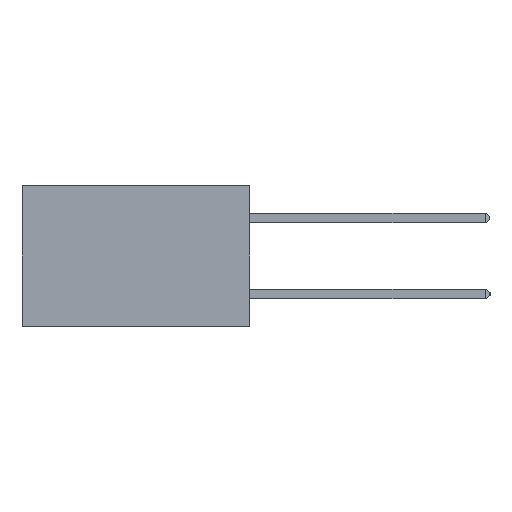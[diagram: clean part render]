
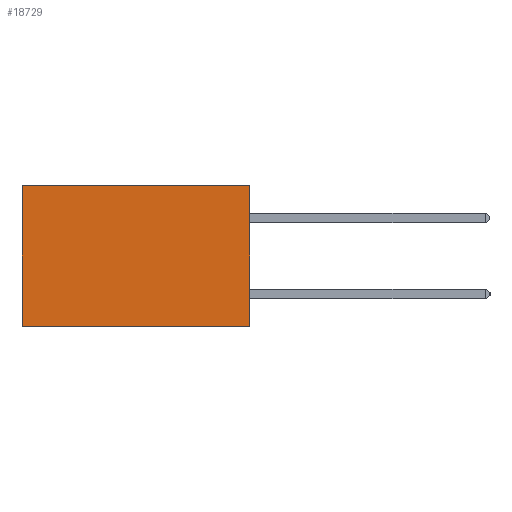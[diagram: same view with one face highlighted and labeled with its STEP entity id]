
A CAD part, left-side view. The second image highlights one B-rep face of the part: STEP entity #18729.
In plain terms, the highlighted planar face has unit normal (-1, 0, 0).
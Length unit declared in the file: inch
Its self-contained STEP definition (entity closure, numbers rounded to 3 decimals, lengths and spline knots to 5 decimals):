
#870 = DIRECTION ( 'NONE',  ( 0., 0., -1. ) ) ;
#1429 = VERTEX_POINT ( 'NONE', #18514 ) ;
#1780 = ORIENTED_EDGE ( 'NONE', *, *, #9348, .T. ) ;
#2032 = VECTOR ( 'NONE', #22287, 39.37008 ) ;
#2166 = VERTEX_POINT ( 'NONE', #12702 ) ;
#5112 = VECTOR ( 'NONE', #22371, 39.37008 ) ;
#5744 = LINE ( 'NONE', #7700, #2032 ) ;
#6310 = CARTESIAN_POINT ( 'NONE',  ( 0.2875, 0., 0. ) ) ;
#6389 = DIRECTION ( 'NONE',  ( 1., 0., 0. ) ) ;
#6594 = CARTESIAN_POINT ( 'NONE',  ( 0.2875, 0., -0.37 ) ) ;
#7700 = CARTESIAN_POINT ( 'NONE',  ( 0.2875, 0., 0. ) ) ;
#7823 = ORIENTED_EDGE ( 'NONE', *, *, #16398, .F. ) ;
#8543 = LINE ( 'NONE', #6594, #5112 ) ;
#9080 = VERTEX_POINT ( 'NONE', #19997 ) ;
#9171 = EDGE_CURVE ( 'NONE', #9080, #1429, #5744, .T. ) ;
#9348 = EDGE_CURVE ( 'NONE', #1429, #2166, #10896, .T. ) ;
#9807 = PLANE ( 'NONE',  #16228 ) ;
#10896 = LINE ( 'NONE', #21007, #22033 ) ;
#12702 = CARTESIAN_POINT ( 'NONE',  ( 0.2875, 0.6, -0.37 ) ) ;
#13511 = ORIENTED_EDGE ( 'NONE', *, *, #9171, .T. ) ;
#13743 = ORIENTED_EDGE ( 'NONE', *, *, #17037, .F. ) ;
#13765 = CARTESIAN_POINT ( 'NONE',  ( 0.2875, 0., 0. ) ) ;
#13851 = DIRECTION ( 'NONE',  ( 0., 0., -1. ) ) ;
#14494 = CARTESIAN_POINT ( 'NONE',  ( 0.2875, 0., -0.37 ) ) ;
#14846 = LINE ( 'NONE', #13765, #22539 ) ;
#16228 = AXIS2_PLACEMENT_3D ( 'NONE', #6310, #6389, #870 ) ;
#16398 = EDGE_CURVE ( 'NONE', #9080, #16684, #14846, .T. ) ;
#16684 = VERTEX_POINT ( 'NONE', #14494 ) ;
#17037 = EDGE_CURVE ( 'NONE', #16684, #2166, #8543, .T. ) ;
#18514 = CARTESIAN_POINT ( 'NONE',  ( 0.2875, 0.6, 0. ) ) ;
#18729 = ADVANCED_FACE ( 'NONE', ( #20716 ), #9807, .F. ) ;
#19171 = DIRECTION ( 'NONE',  ( 0., 0., -1. ) ) ;
#19997 = CARTESIAN_POINT ( 'NONE',  ( 0.2875, 0., 0. ) ) ;
#20716 = FACE_OUTER_BOUND ( 'NONE', #21560, .T. ) ;
#21007 = CARTESIAN_POINT ( 'NONE',  ( 0.2875, 0.6, 0. ) ) ;
#21560 = EDGE_LOOP ( 'NONE', ( #1780, #13743, #7823, #13511 ) ) ;
#22033 = VECTOR ( 'NONE', #19171, 39.37008 ) ;
#22287 = DIRECTION ( 'NONE',  ( 0., 1., 0. ) ) ;
#22371 = DIRECTION ( 'NONE',  ( 0., 1., 0. ) ) ;
#22539 = VECTOR ( 'NONE', #13851, 39.37008 ) ;
